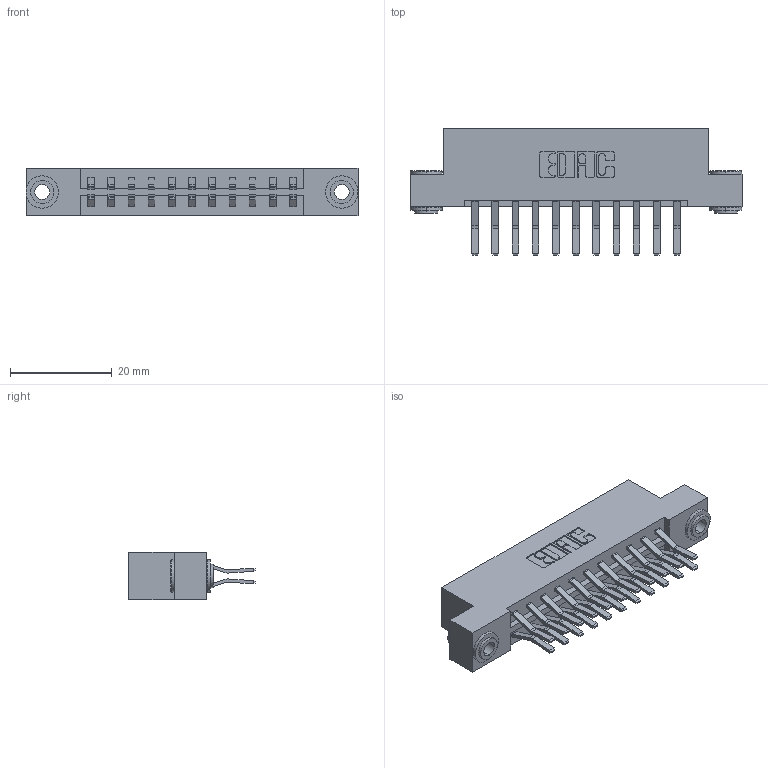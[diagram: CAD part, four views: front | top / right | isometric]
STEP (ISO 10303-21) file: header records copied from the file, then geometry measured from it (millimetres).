
FILE_DESCRIPTION (( 'STEP AP203' ), '1' );
FILE_NAME ('833-022-560-203.STEP', '2020-06-01T18:27:02', ( '' ), ( '' ), 'SwSTEP 2.0', 'SolidWorks 2020', '' );
FILE_SCHEMA (( 'CONFIG_CONTROL_DESIGN' ));
Length unit declared in the file: inch
Products named in the file (4): 833-022-560-203; 345-250-002_345-250-002-102; 833 Part_Flush - .156 Dia - TH; 345-292-001_560 Tail
Assembly tree (25 placements, depth 2):
  833-022-560-203
    833 Part_Flush - .156 Dia - TH
    345-292-001_560 Tail  x22
    345-250-002_345-250-002-102  x2
Bounding box: 65.13 x 24.78 x 9.4 mm (x, y, z)
Volume: 6522.6 mm3; surface area: 8010.5 mm2
Topology: 25 solids, 25 shells, 1340 faces, 3929 edges, 2586 vertices
Faces by surface type: plane 872, cylinder 460, cone 8
Entity records: 11824 total; most frequent: CARTESIAN_POINT 1973, ORIENTED_EDGE 1902, DIRECTION 1777, EDGE_CURVE 951, LINE 795, VECTOR 795, VERTEX_POINT 630, AXIS2_PLACEMENT_3D 491
